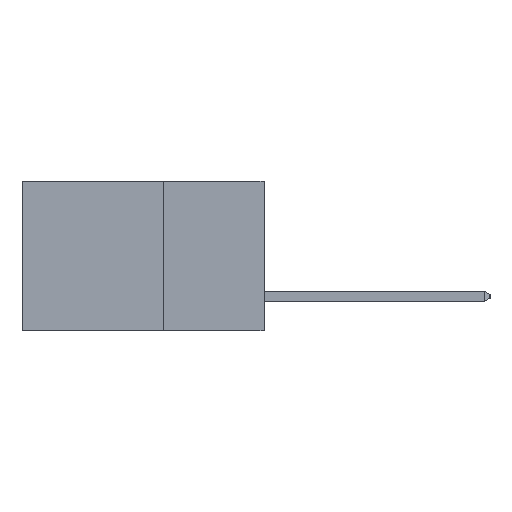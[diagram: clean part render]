
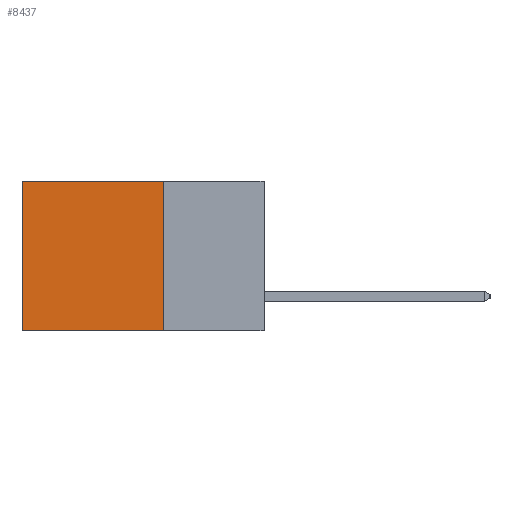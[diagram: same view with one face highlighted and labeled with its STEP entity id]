
A CAD part, left-side view. The second image highlights one B-rep face of the part: STEP entity #8437.
In plain terms, the highlighted planar face has unit normal (-1, 0, 0).
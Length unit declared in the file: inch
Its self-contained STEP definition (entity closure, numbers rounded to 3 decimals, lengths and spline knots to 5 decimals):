
#119 = FACE_OUTER_BOUND ( 'NONE', #15044, .T. ) ;
#548 = VERTEX_POINT ( 'NONE', #3594 ) ;
#1187 = VERTEX_POINT ( 'NONE', #14829 ) ;
#1334 = CARTESIAN_POINT ( 'NONE',  ( 0.2615, 0.25, -0.37 ) ) ;
#1751 = AXIS2_PLACEMENT_3D ( 'NONE', #1334, #3371, #17519 ) ;
#1853 = ORIENTED_EDGE ( 'NONE', *, *, #4784, .T. ) ;
#3371 = DIRECTION ( 'NONE',  ( 1., 0., 0. ) ) ;
#3594 = CARTESIAN_POINT ( 'NONE',  ( 0.2615, 0.6, 0. ) ) ;
#4784 = EDGE_CURVE ( 'NONE', #1187, #548, #25714, .T. ) ;
#6204 = EDGE_CURVE ( 'NONE', #548, #8846, #7248, .T. ) ;
#6636 = VECTOR ( 'NONE', #12208, 39.37008 ) ;
#7029 = DIRECTION ( 'NONE',  ( 0., 1., 0. ) ) ;
#7248 = LINE ( 'NONE', #12251, #6636 ) ;
#8181 = CARTESIAN_POINT ( 'NONE',  ( 0.2615, 0.25, -0.37 ) ) ;
#8437 = ADVANCED_FACE ( 'NONE', ( #119 ), #25328, .F. ) ;
#8846 = VERTEX_POINT ( 'NONE', #18695 ) ;
#9448 = VECTOR ( 'NONE', #19791, 39.37008 ) ;
#10034 = VERTEX_POINT ( 'NONE', #8181 ) ;
#10365 = CARTESIAN_POINT ( 'NONE',  ( 0.2615, 0.25, 0. ) ) ;
#10712 = DIRECTION ( 'NONE',  ( 0., 1., 0. ) ) ;
#11001 = VECTOR ( 'NONE', #7029, 39.37008 ) ;
#11100 = VECTOR ( 'NONE', #10712, 39.37008 ) ;
#12208 = DIRECTION ( 'NONE',  ( 0., 0., -1. ) ) ;
#12251 = CARTESIAN_POINT ( 'NONE',  ( 0.2615, 0.6, -0.37 ) ) ;
#14254 = EDGE_CURVE ( 'NONE', #10034, #8846, #21026, .T. ) ;
#14829 = CARTESIAN_POINT ( 'NONE',  ( 0.2615, 0.25, 0. ) ) ;
#14879 = LINE ( 'NONE', #17799, #9448 ) ;
#15044 = EDGE_LOOP ( 'NONE', ( #16643, #18898, #24516, #1853 ) ) ;
#16643 = ORIENTED_EDGE ( 'NONE', *, *, #6204, .T. ) ;
#17519 = DIRECTION ( 'NONE',  ( 0., 0., -1. ) ) ;
#17799 = CARTESIAN_POINT ( 'NONE',  ( 0.2615, 0.25, -0.37 ) ) ;
#18314 = EDGE_CURVE ( 'NONE', #1187, #10034, #14879, .T. ) ;
#18695 = CARTESIAN_POINT ( 'NONE',  ( 0.2615, 0.6, -0.37 ) ) ;
#18898 = ORIENTED_EDGE ( 'NONE', *, *, #14254, .F. ) ;
#19081 = CARTESIAN_POINT ( 'NONE',  ( 0.2615, 0.25, -0.37 ) ) ;
#19791 = DIRECTION ( 'NONE',  ( 0., 0., -1. ) ) ;
#21026 = LINE ( 'NONE', #19081, #11001 ) ;
#24516 = ORIENTED_EDGE ( 'NONE', *, *, #18314, .F. ) ;
#25328 = PLANE ( 'NONE',  #1751 ) ;
#25714 = LINE ( 'NONE', #10365, #11100 ) ;
